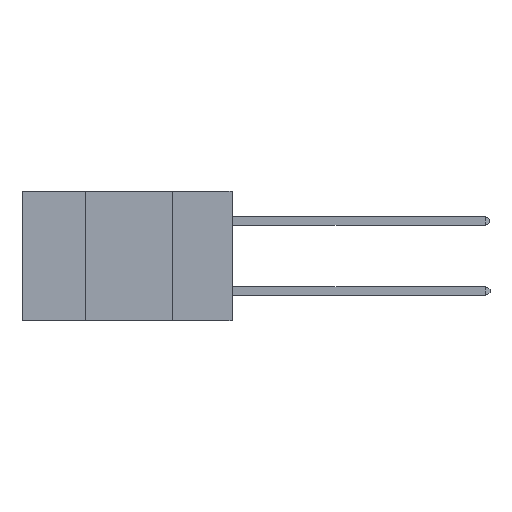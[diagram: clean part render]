
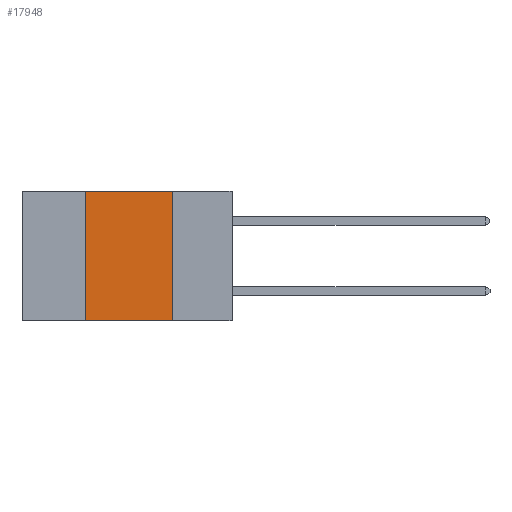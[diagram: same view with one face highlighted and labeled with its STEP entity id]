
A CAD part, left-side view. The second image highlights one B-rep face of the part: STEP entity #17948.
In plain terms, the highlighted planar face has unit normal (-1, 0, 0).
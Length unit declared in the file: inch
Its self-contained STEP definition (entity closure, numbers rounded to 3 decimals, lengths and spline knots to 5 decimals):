
#352 = DIRECTION ( 'NONE',  ( 0., 0., -1. ) ) ;
#2204 = ORIENTED_EDGE ( 'NONE', *, *, #15075, .F. ) ;
#2362 = CARTESIAN_POINT ( 'NONE',  ( 0., 0.6, 0. ) ) ;
#2397 = CARTESIAN_POINT ( 'NONE',  ( 0., 0.42, -0.37 ) ) ;
#3436 = CARTESIAN_POINT ( 'NONE',  ( 0., 0.17, 0. ) ) ;
#3461 = EDGE_CURVE ( 'NONE', #14262, #18322, #10743, .T. ) ;
#3490 = CARTESIAN_POINT ( 'NONE',  ( 0., 0.6, -0.37 ) ) ;
#4089 = VERTEX_POINT ( 'NONE', #4304 ) ;
#4163 = DIRECTION ( 'NONE',  ( 0., 0., -1. ) ) ;
#4304 = CARTESIAN_POINT ( 'NONE',  ( 0., 0.17, -0.37 ) ) ;
#4609 = FACE_OUTER_BOUND ( 'NONE', #20607, .T. ) ;
#4661 = ORIENTED_EDGE ( 'NONE', *, *, #11638, .F. ) ;
#4671 = LINE ( 'NONE', #13977, #8679 ) ;
#5408 = DIRECTION ( 'NONE',  ( 0., 0., 1. ) ) ;
#6207 = VECTOR ( 'NONE', #15659, 39.37008 ) ;
#6888 = ORIENTED_EDGE ( 'NONE', *, *, #3461, .F. ) ;
#8196 = AXIS2_PLACEMENT_3D ( 'NONE', #2362, #14467, #4163 ) ;
#8679 = VECTOR ( 'NONE', #5408, 39.37008 ) ;
#9766 = VECTOR ( 'NONE', #15533, 39.37008 ) ;
#9803 = ORIENTED_EDGE ( 'NONE', *, *, #10910, .T. ) ;
#10743 = LINE ( 'NONE', #15995, #6207 ) ;
#10910 = EDGE_CURVE ( 'NONE', #19782, #4089, #17781, .T. ) ;
#11638 = EDGE_CURVE ( 'NONE', #19782, #14262, #4671, .T. ) ;
#12777 = PLANE ( 'NONE',  #8196 ) ;
#13977 = CARTESIAN_POINT ( 'NONE',  ( 0., 0.42, 0. ) ) ;
#14262 = VERTEX_POINT ( 'NONE', #17296 ) ;
#14467 = DIRECTION ( 'NONE',  ( 1., 0., 0. ) ) ;
#15075 = EDGE_CURVE ( 'NONE', #18322, #4089, #21574, .T. ) ;
#15533 = DIRECTION ( 'NONE',  ( 0., -1., 0. ) ) ;
#15659 = DIRECTION ( 'NONE',  ( 0., -1., 0. ) ) ;
#15995 = CARTESIAN_POINT ( 'NONE',  ( 0., 0.6, 0. ) ) ;
#17296 = CARTESIAN_POINT ( 'NONE',  ( 0., 0.42, 0. ) ) ;
#17781 = LINE ( 'NONE', #3490, #9766 ) ;
#17948 = ADVANCED_FACE ( 'NONE', ( #4609 ), #12777, .F. ) ;
#18322 = VERTEX_POINT ( 'NONE', #3436 ) ;
#19782 = VERTEX_POINT ( 'NONE', #2397 ) ;
#20607 = EDGE_LOOP ( 'NONE', ( #2204, #6888, #4661, #9803 ) ) ;
#21014 = CARTESIAN_POINT ( 'NONE',  ( 0., 0.17, 0. ) ) ;
#21040 = VECTOR ( 'NONE', #352, 39.37008 ) ;
#21574 = LINE ( 'NONE', #21014, #21040 ) ;
